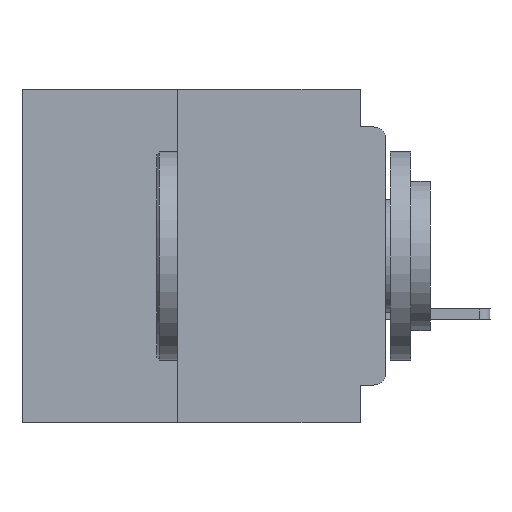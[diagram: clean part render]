
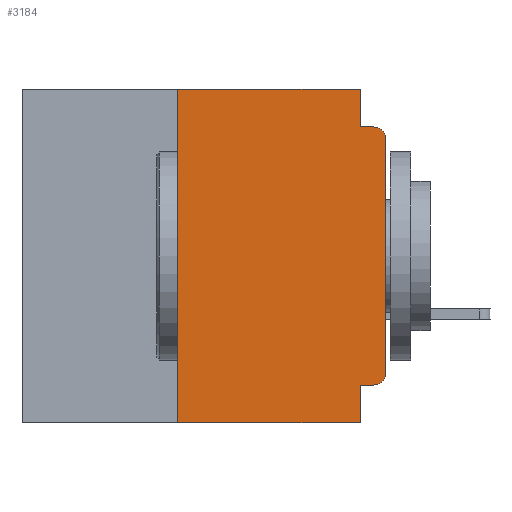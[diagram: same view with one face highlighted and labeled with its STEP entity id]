
A CAD part, left-side view. The second image highlights one B-rep face of the part: STEP entity #3184.
In plain terms, the highlighted planar face has unit normal (-1, 0, 0).
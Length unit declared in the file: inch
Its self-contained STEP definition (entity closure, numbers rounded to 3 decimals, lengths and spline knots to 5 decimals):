
#67 = CARTESIAN_POINT ( 'NONE',  ( 0., 0.031, 0. ) ) ;
#616 = EDGE_CURVE ( 'NONE', #58798, #16918, #32318, .T. ) ;
#1075 = VERTEX_POINT ( 'NONE', #26296 ) ;
#1165 = LINE ( 'NONE', #24982, #12162 ) ;
#1667 = DIRECTION ( 'NONE',  ( 0., 0., 1. ) ) ;
#1720 = ORIENTED_EDGE ( 'NONE', *, *, #54976, .F. ) ;
#3184 = ADVANCED_FACE ( 'NONE', ( #22572 ), #11572, .F. ) ;
#3228 = EDGE_CURVE ( 'NONE', #20838, #37821, #33487, .T. ) ;
#4799 = DIRECTION ( 'NONE',  ( 0., 0., -1. ) ) ;
#5392 = LINE ( 'NONE', #53015, #22226 ) ;
#10776 = CARTESIAN_POINT ( 'NONE',  ( 0., 0.031, -0.4 ) ) ;
#11192 = CARTESIAN_POINT ( 'NONE',  ( 0., 0., -0.045 ) ) ;
#11572 = PLANE ( 'NONE',  #38852 ) ;
#11838 = CARTESIAN_POINT ( 'NONE',  ( 0., 0.437, 0. ) ) ;
#12162 = VECTOR ( 'NONE', #1667, 39.37008 ) ;
#12245 = DIRECTION ( 'NONE',  ( 0., -1., 0. ) ) ;
#12728 = CARTESIAN_POINT ( 'NONE',  ( 0., 0.25, -0.4 ) ) ;
#12933 = CARTESIAN_POINT ( 'NONE',  ( 0., 0.015, -0.34 ) ) ;
#14196 = EDGE_CURVE ( 'NONE', #1075, #45612, #22299, .T. ) ;
#14716 = CARTESIAN_POINT ( 'NONE',  ( 0., 0., -0.34 ) ) ;
#15489 = DIRECTION ( 'NONE',  ( 0., 0., -1. ) ) ;
#15900 = DIRECTION ( 'NONE',  ( 0., -1., 0. ) ) ;
#16916 = CARTESIAN_POINT ( 'NONE',  ( 0., 0.031, -0.4 ) ) ;
#16918 = VERTEX_POINT ( 'NONE', #40400 ) ;
#17645 = DIRECTION ( 'NONE',  ( 0., 0., -1. ) ) ;
#18222 = CIRCLE ( 'NONE', #53863, 0.015 ) ;
#18553 = ORIENTED_EDGE ( 'NONE', *, *, #29984, .F. ) ;
#18944 = CARTESIAN_POINT ( 'NONE',  ( 0., 0., 0. ) ) ;
#19005 = EDGE_CURVE ( 'NONE', #32352, #21842, #18222, .T. ) ;
#20838 = VERTEX_POINT ( 'NONE', #12728 ) ;
#21842 = VERTEX_POINT ( 'NONE', #14716 ) ;
#22226 = VECTOR ( 'NONE', #57578, 39.37008 ) ;
#22295 = CARTESIAN_POINT ( 'NONE',  ( 0., 0.031, -0.355 ) ) ;
#22299 = LINE ( 'NONE', #11192, #57490 ) ;
#22572 = FACE_OUTER_BOUND ( 'NONE', #47739, .T. ) ;
#22666 = ORIENTED_EDGE ( 'NONE', *, *, #3228, .T. ) ;
#22702 = DIRECTION ( 'NONE',  ( -1., 0., 0. ) ) ;
#24635 = CARTESIAN_POINT ( 'NONE',  ( 0., 0.015, -0.355 ) ) ;
#24982 = CARTESIAN_POINT ( 'NONE',  ( 0., 0.25, -0.4 ) ) ;
#25529 = ORIENTED_EDGE ( 'NONE', *, *, #29569, .T. ) ;
#26296 = CARTESIAN_POINT ( 'NONE',  ( 0., 0.031, -0.045 ) ) ;
#27646 = VECTOR ( 'NONE', #4799, 39.37008 ) ;
#29432 = EDGE_CURVE ( 'NONE', #46410, #45612, #42870, .T. ) ;
#29569 = EDGE_CURVE ( 'NONE', #21842, #46410, #47797, .T. ) ;
#29984 = EDGE_CURVE ( 'NONE', #56273, #37821, #35620, .T. ) ;
#30544 = ORIENTED_EDGE ( 'NONE', *, *, #29432, .T. ) ;
#30905 = DIRECTION ( 'NONE',  ( 0., 0., -1. ) ) ;
#30945 = ORIENTED_EDGE ( 'NONE', *, *, #46073, .F. ) ;
#31111 = CARTESIAN_POINT ( 'NONE',  ( 0., 0.437, -0.4 ) ) ;
#32318 = LINE ( 'NONE', #11838, #38747 ) ;
#32352 = VERTEX_POINT ( 'NONE', #24635 ) ;
#32901 = CARTESIAN_POINT ( 'NONE',  ( 0., 0.437, 0. ) ) ;
#33487 = LINE ( 'NONE', #31111, #59180 ) ;
#35141 = EDGE_CURVE ( 'NONE', #20838, #58798, #1165, .T. ) ;
#35586 = ORIENTED_EDGE ( 'NONE', *, *, #14196, .F. ) ;
#35620 = LINE ( 'NONE', #10776, #58441 ) ;
#37460 = AXIS2_PLACEMENT_3D ( 'NONE', #50252, #22702, #54858 ) ;
#37821 = VERTEX_POINT ( 'NONE', #16916 ) ;
#38747 = VECTOR ( 'NONE', #12245, 39.37008 ) ;
#38852 = AXIS2_PLACEMENT_3D ( 'NONE', #32901, #55785, #30905 ) ;
#40400 = CARTESIAN_POINT ( 'NONE',  ( 0., 0.031, 0. ) ) ;
#42870 = CIRCLE ( 'NONE', #37460, 0.015 ) ;
#45350 = DIRECTION ( 'NONE',  ( -1., 0., 0. ) ) ;
#45612 = VERTEX_POINT ( 'NONE', #49471 ) ;
#46073 = EDGE_CURVE ( 'NONE', #32352, #56273, #5392, .T. ) ;
#46403 = CARTESIAN_POINT ( 'NONE',  ( 0., 0., -0.06 ) ) ;
#46410 = VERTEX_POINT ( 'NONE', #46403 ) ;
#46430 = DIRECTION ( 'NONE',  ( 0., -1., 0. ) ) ;
#47739 = EDGE_LOOP ( 'NONE', ( #25529, #30544, #35586, #1720, #50766, #49814, #22666, #18553, #30945, #50010 ) ) ;
#47797 = LINE ( 'NONE', #18944, #59927 ) ;
#49471 = CARTESIAN_POINT ( 'NONE',  ( 0., 0.015, -0.045 ) ) ;
#49814 = ORIENTED_EDGE ( 'NONE', *, *, #35141, .F. ) ;
#50010 = ORIENTED_EDGE ( 'NONE', *, *, #19005, .T. ) ;
#50252 = CARTESIAN_POINT ( 'NONE',  ( 0., 0.015, -0.06 ) ) ;
#50766 = ORIENTED_EDGE ( 'NONE', *, *, #616, .F. ) ;
#50829 = CARTESIAN_POINT ( 'NONE',  ( 0., 0.25, 0. ) ) ;
#53015 = CARTESIAN_POINT ( 'NONE',  ( 0., 0., -0.355 ) ) ;
#53863 = AXIS2_PLACEMENT_3D ( 'NONE', #12933, #45350, #17645 ) ;
#54858 = DIRECTION ( 'NONE',  ( 0., 0., -1. ) ) ;
#54905 = LINE ( 'NONE', #67, #27646 ) ;
#54976 = EDGE_CURVE ( 'NONE', #16918, #1075, #54905, .T. ) ;
#55617 = DIRECTION ( 'NONE',  ( 0., 0., 1. ) ) ;
#55785 = DIRECTION ( 'NONE',  ( 1., 0., 0. ) ) ;
#56273 = VERTEX_POINT ( 'NONE', #22295 ) ;
#57490 = VECTOR ( 'NONE', #15900, 39.37008 ) ;
#57578 = DIRECTION ( 'NONE',  ( 0., 1., 0. ) ) ;
#58441 = VECTOR ( 'NONE', #15489, 39.37008 ) ;
#58798 = VERTEX_POINT ( 'NONE', #50829 ) ;
#59180 = VECTOR ( 'NONE', #46430, 39.37008 ) ;
#59927 = VECTOR ( 'NONE', #55617, 39.37008 ) ;
